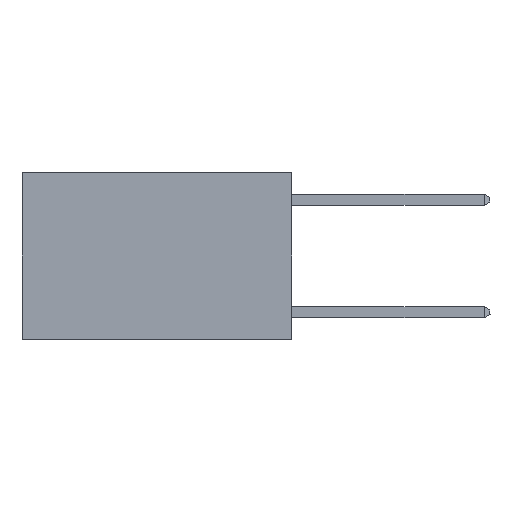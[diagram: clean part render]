
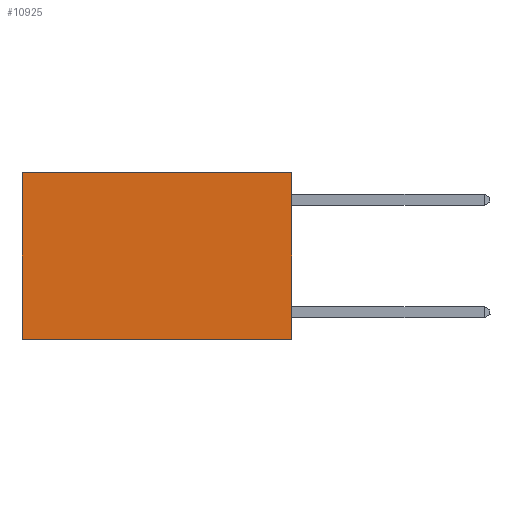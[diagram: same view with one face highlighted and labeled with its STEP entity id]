
A CAD part, left-side view. The second image highlights one B-rep face of the part: STEP entity #10925.
In plain terms, the highlighted planar face has unit normal (-1, 0, 0).
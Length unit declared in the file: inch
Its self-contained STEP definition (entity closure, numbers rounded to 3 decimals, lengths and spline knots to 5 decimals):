
#1140 = EDGE_CURVE ( 'NONE', #12787, #3623, #11667, .T. ) ;
#1367 = CARTESIAN_POINT ( 'NONE',  ( 0.2625, 0.6, 0. ) ) ;
#1409 = CARTESIAN_POINT ( 'NONE',  ( 0.2625, 0., -0.37 ) ) ;
#1555 = FACE_OUTER_BOUND ( 'NONE', #11321, .T. ) ;
#2604 = CARTESIAN_POINT ( 'NONE',  ( 0.2625, 0., 0. ) ) ;
#3623 = VERTEX_POINT ( 'NONE', #5214 ) ;
#4232 = VERTEX_POINT ( 'NONE', #4771 ) ;
#4476 = DIRECTION ( 'NONE',  ( 0., 0., -1. ) ) ;
#4771 = CARTESIAN_POINT ( 'NONE',  ( 0.2625, 0., 0. ) ) ;
#4955 = PLANE ( 'NONE',  #22051 ) ;
#5214 = CARTESIAN_POINT ( 'NONE',  ( 0.2625, 0.6, -0.37 ) ) ;
#6795 = CARTESIAN_POINT ( 'NONE',  ( 0.2625, 0., 0. ) ) ;
#6805 = VECTOR ( 'NONE', #21072, 39.37008 ) ;
#7125 = CARTESIAN_POINT ( 'NONE',  ( 0.2625, 0.6, 0. ) ) ;
#7652 = VECTOR ( 'NONE', #21399, 39.37008 ) ;
#8685 = DIRECTION ( 'NONE',  ( 0., 0., -1. ) ) ;
#10925 = ADVANCED_FACE ( 'NONE', ( #1555 ), #4955, .F. ) ;
#11321 = EDGE_LOOP ( 'NONE', ( #14123, #14144, #14367, #14654 ) ) ;
#11622 = VECTOR ( 'NONE', #18011, 39.37008 ) ;
#11667 = LINE ( 'NONE', #7125, #11622 ) ;
#11980 = VECTOR ( 'NONE', #4476, 39.37008 ) ;
#12787 = VERTEX_POINT ( 'NONE', #1367 ) ;
#13606 = EDGE_CURVE ( 'NONE', #18629, #3623, #21019, .T. ) ;
#14123 = ORIENTED_EDGE ( 'NONE', *, *, #1140, .T. ) ;
#14144 = ORIENTED_EDGE ( 'NONE', *, *, #13606, .F. ) ;
#14152 = EDGE_CURVE ( 'NONE', #4232, #12787, #17907, .T. ) ;
#14367 = ORIENTED_EDGE ( 'NONE', *, *, #16717, .F. ) ;
#14654 = ORIENTED_EDGE ( 'NONE', *, *, #14152, .T. ) ;
#16717 = EDGE_CURVE ( 'NONE', #4232, #18629, #21130, .T. ) ;
#17907 = LINE ( 'NONE', #19772, #7652 ) ;
#18011 = DIRECTION ( 'NONE',  ( 0., 0., -1. ) ) ;
#18629 = VERTEX_POINT ( 'NONE', #1409 ) ;
#19403 = DIRECTION ( 'NONE',  ( 1., 0., 0. ) ) ;
#19436 = CARTESIAN_POINT ( 'NONE',  ( 0.2625, 0., -0.37 ) ) ;
#19772 = CARTESIAN_POINT ( 'NONE',  ( 0.2625, 0., 0. ) ) ;
#21019 = LINE ( 'NONE', #19436, #6805 ) ;
#21072 = DIRECTION ( 'NONE',  ( 0., 1., 0. ) ) ;
#21130 = LINE ( 'NONE', #2604, #11980 ) ;
#21399 = DIRECTION ( 'NONE',  ( 0., 1., 0. ) ) ;
#22051 = AXIS2_PLACEMENT_3D ( 'NONE', #6795, #19403, #8685 ) ;
